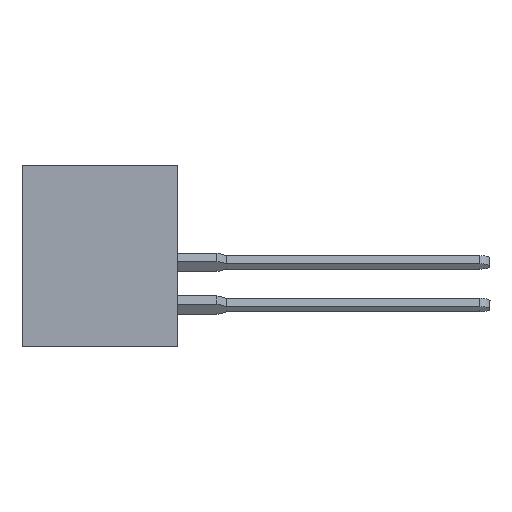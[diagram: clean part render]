
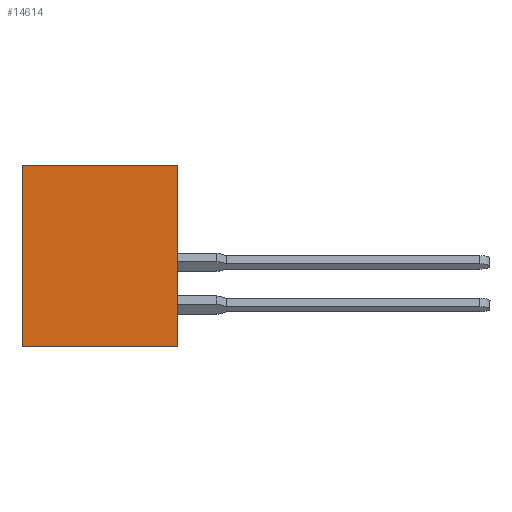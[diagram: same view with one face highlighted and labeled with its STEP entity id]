
A CAD part, left-side view. The second image highlights one B-rep face of the part: STEP entity #14614.
In plain terms, the highlighted planar face has unit normal (-1, 0, 0).
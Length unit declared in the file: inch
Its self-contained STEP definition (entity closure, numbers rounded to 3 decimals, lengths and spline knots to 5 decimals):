
#609 = VECTOR ( 'NONE', #18285, 39.37008 ) ;
#1273 = LINE ( 'NONE', #24435, #609 ) ;
#1967 = DIRECTION ( 'NONE',  ( 0., 0., -1. ) ) ;
#3374 = LINE ( 'NONE', #8500, #13633 ) ;
#5729 = ORIENTED_EDGE ( 'NONE', *, *, #25124, .F. ) ;
#7003 = AXIS2_PLACEMENT_3D ( 'NONE', #8847, #27340, #1967 ) ;
#7503 = EDGE_LOOP ( 'NONE', ( #8638, #5729, #10614, #21201 ) ) ;
#8150 = CARTESIAN_POINT ( 'NONE',  ( 0., 0., -0.531 ) ) ;
#8500 = CARTESIAN_POINT ( 'NONE',  ( 0., 0.453, 0. ) ) ;
#8638 = ORIENTED_EDGE ( 'NONE', *, *, #9852, .T. ) ;
#8847 = CARTESIAN_POINT ( 'NONE',  ( 0., 0.453, 0. ) ) ;
#9781 = LINE ( 'NONE', #10278, #19991 ) ;
#9852 = EDGE_CURVE ( 'NONE', #22225, #14127, #1273, .T. ) ;
#10103 = FACE_OUTER_BOUND ( 'NONE', #7503, .T. ) ;
#10278 = CARTESIAN_POINT ( 'NONE',  ( 0., 0.453, 0. ) ) ;
#10614 = ORIENTED_EDGE ( 'NONE', *, *, #23246, .F. ) ;
#11031 = VERTEX_POINT ( 'NONE', #12611 ) ;
#12611 = CARTESIAN_POINT ( 'NONE',  ( 0., 0.453, 0. ) ) ;
#12711 = VECTOR ( 'NONE', #20141, 39.37008 ) ;
#13633 = VECTOR ( 'NONE', #23298, 39.37008 ) ;
#14041 = CARTESIAN_POINT ( 'NONE',  ( 0., 0.453, -0.531 ) ) ;
#14127 = VERTEX_POINT ( 'NONE', #15239 ) ;
#14614 = ADVANCED_FACE ( 'NONE', ( #10103 ), #25890, .F. ) ;
#15239 = CARTESIAN_POINT ( 'NONE',  ( 0., 0., 0. ) ) ;
#17330 = LINE ( 'NONE', #14041, #12711 ) ;
#18285 = DIRECTION ( 'NONE',  ( 0., 0., 1. ) ) ;
#19991 = VECTOR ( 'NONE', #23013, 39.37008 ) ;
#20141 = DIRECTION ( 'NONE',  ( 0., -1., 0. ) ) ;
#21201 = ORIENTED_EDGE ( 'NONE', *, *, #23627, .T. ) ;
#22225 = VERTEX_POINT ( 'NONE', #8150 ) ;
#23013 = DIRECTION ( 'NONE',  ( 0., 0., 1. ) ) ;
#23114 = CARTESIAN_POINT ( 'NONE',  ( 0., 0.453, -0.531 ) ) ;
#23246 = EDGE_CURVE ( 'NONE', #25217, #11031, #9781, .T. ) ;
#23298 = DIRECTION ( 'NONE',  ( 0., -1., 0. ) ) ;
#23627 = EDGE_CURVE ( 'NONE', #25217, #22225, #17330, .T. ) ;
#24435 = CARTESIAN_POINT ( 'NONE',  ( 0., 0., 0. ) ) ;
#25124 = EDGE_CURVE ( 'NONE', #11031, #14127, #3374, .T. ) ;
#25217 = VERTEX_POINT ( 'NONE', #23114 ) ;
#25890 = PLANE ( 'NONE',  #7003 ) ;
#27340 = DIRECTION ( 'NONE',  ( 1., 0., 0. ) ) ;
